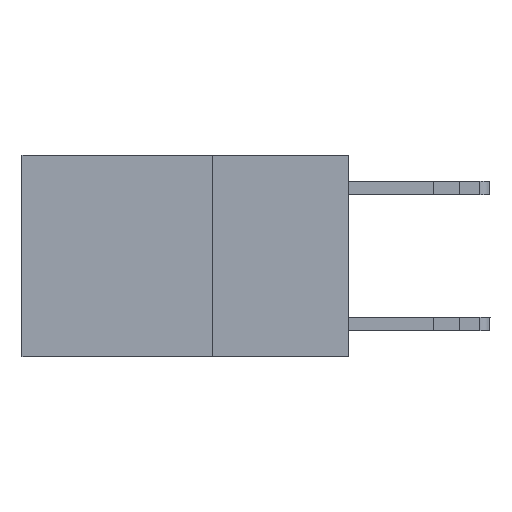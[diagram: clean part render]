
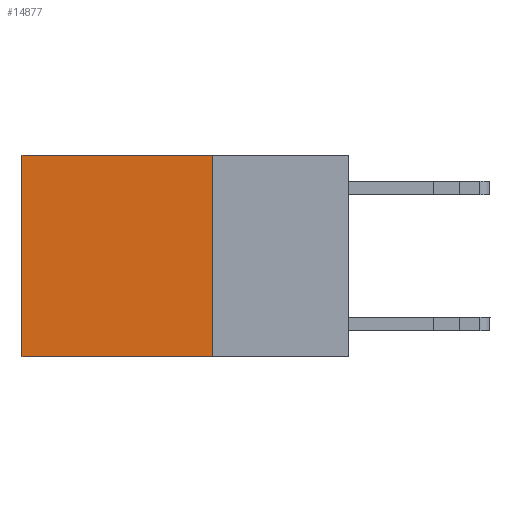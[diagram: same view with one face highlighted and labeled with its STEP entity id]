
A CAD part, left-side view. The second image highlights one B-rep face of the part: STEP entity #14877.
In plain terms, the highlighted planar face has unit normal (-1, 0, 0).
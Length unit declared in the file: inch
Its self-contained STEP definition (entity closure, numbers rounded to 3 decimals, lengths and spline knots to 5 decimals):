
#264 = PLANE ( 'NONE',  #3894 ) ;
#2282 = CARTESIAN_POINT ( 'NONE',  ( 0.2625, 0.25, 0. ) ) ;
#2315 = VERTEX_POINT ( 'NONE', #21787 ) ;
#2591 = DIRECTION ( 'NONE',  ( 0., 0., -1. ) ) ;
#2803 = LINE ( 'NONE', #14819, #10161 ) ;
#3894 = AXIS2_PLACEMENT_3D ( 'NONE', #2282, #14476, #21062 ) ;
#5160 = ORIENTED_EDGE ( 'NONE', *, *, #10648, .T. ) ;
#5941 = DIRECTION ( 'NONE',  ( 0., 1., 0. ) ) ;
#6223 = CARTESIAN_POINT ( 'NONE',  ( 0.2625, 0.25, 0. ) ) ;
#8276 = VECTOR ( 'NONE', #10506, 39.37008 ) ;
#9098 = CARTESIAN_POINT ( 'NONE',  ( 0.2625, 0.25, -0.37 ) ) ;
#10161 = VECTOR ( 'NONE', #2591, 39.37008 ) ;
#10506 = DIRECTION ( 'NONE',  ( 0., 1., 0. ) ) ;
#10648 = EDGE_CURVE ( 'NONE', #12972, #2315, #20538, .T. ) ;
#11073 = CARTESIAN_POINT ( 'NONE',  ( 0.2625, 0.25, -0.37 ) ) ;
#11620 = EDGE_LOOP ( 'NONE', ( #14699, #16869, #17442, #5160 ) ) ;
#12178 = CARTESIAN_POINT ( 'NONE',  ( 0.2625, 0.6, -0.37 ) ) ;
#12972 = VERTEX_POINT ( 'NONE', #6223 ) ;
#13137 = EDGE_CURVE ( 'NONE', #2315, #17851, #2803, .T. ) ;
#13282 = VECTOR ( 'NONE', #5941, 39.37008 ) ;
#13524 = FACE_OUTER_BOUND ( 'NONE', #11620, .T. ) ;
#14476 = DIRECTION ( 'NONE',  ( 1., 0., 0. ) ) ;
#14569 = DIRECTION ( 'NONE',  ( 0., 0., -1. ) ) ;
#14699 = ORIENTED_EDGE ( 'NONE', *, *, #13137, .T. ) ;
#14819 = CARTESIAN_POINT ( 'NONE',  ( 0.2625, 0.6, 0. ) ) ;
#14877 = ADVANCED_FACE ( 'NONE', ( #13524 ), #264, .F. ) ;
#14936 = VERTEX_POINT ( 'NONE', #11073 ) ;
#16869 = ORIENTED_EDGE ( 'NONE', *, *, #17099, .F. ) ;
#17099 = EDGE_CURVE ( 'NONE', #14936, #17851, #19297, .T. ) ;
#17342 = CARTESIAN_POINT ( 'NONE',  ( 0.2625, 0.25, 0. ) ) ;
#17442 = ORIENTED_EDGE ( 'NONE', *, *, #21766, .F. ) ;
#17851 = VERTEX_POINT ( 'NONE', #12178 ) ;
#19062 = LINE ( 'NONE', #19814, #19205 ) ;
#19205 = VECTOR ( 'NONE', #14569, 39.37008 ) ;
#19297 = LINE ( 'NONE', #9098, #8276 ) ;
#19814 = CARTESIAN_POINT ( 'NONE',  ( 0.2625, 0.25, 0. ) ) ;
#20538 = LINE ( 'NONE', #17342, #13282 ) ;
#21062 = DIRECTION ( 'NONE',  ( 0., 0., -1. ) ) ;
#21766 = EDGE_CURVE ( 'NONE', #12972, #14936, #19062, .T. ) ;
#21787 = CARTESIAN_POINT ( 'NONE',  ( 0.2625, 0.6, 0. ) ) ;
